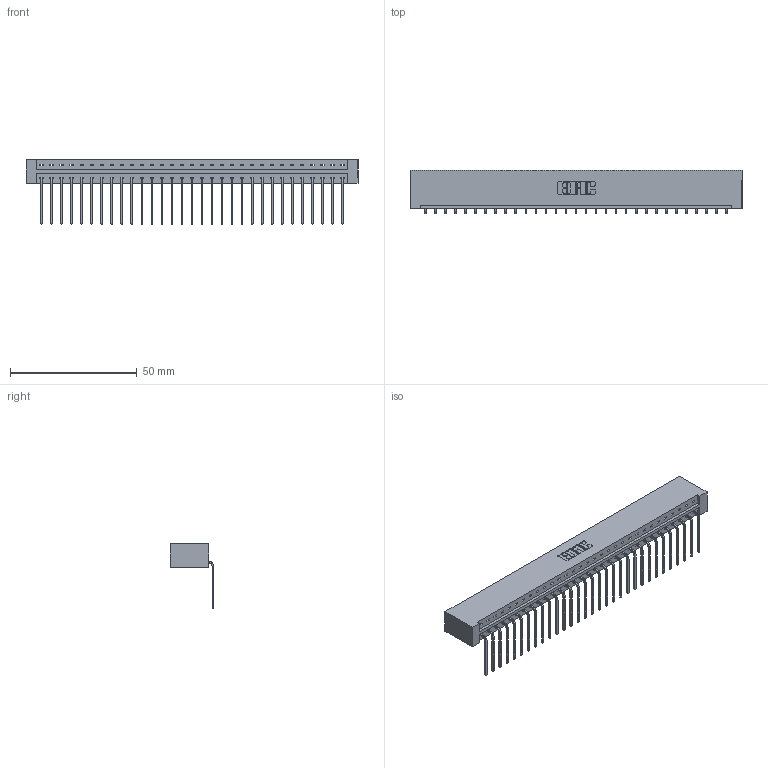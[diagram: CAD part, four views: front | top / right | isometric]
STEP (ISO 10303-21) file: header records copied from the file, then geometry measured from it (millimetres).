
FILE_DESCRIPTION (( 'STEP AP203' ), '1' );
FILE_NAME ('833-031-559-101.STEP', '2020-06-02T16:06:27', ( '' ), ( '' ), 'SwSTEP 2.0', 'SolidWorks 2020', '' );
FILE_SCHEMA (( 'CONFIG_CONTROL_DESIGN' ));
Length unit declared in the file: inch
Products named in the file (3): 833 Part_Lugless; 833-031-559-101; 345-292-001_558 559 Tail - 1
Assembly tree (32 placements, depth 2):
  833-031-559-101
    833 Part_Lugless
    345-292-001_558 559 Tail - 1  x31
Bounding box: 131.09 x 17.09 x 25.53 mm (x, y, z)
Volume: 13812.7 mm3; surface area: 15463 mm2
Topology: 32 solids, 32 shells, 1966 faces, 5929 edges, 3910 vertices
Faces by surface type: plane 1430, cylinder 536
Entity records: 20181 total; most frequent: CARTESIAN_POINT 3491, ORIENTED_EDGE 3458, DIRECTION 2959, EDGE_CURVE 1729, VECTOR 1609, LINE 1609, VERTEX_POINT 1150, AXIS2_PLACEMENT_3D 675
